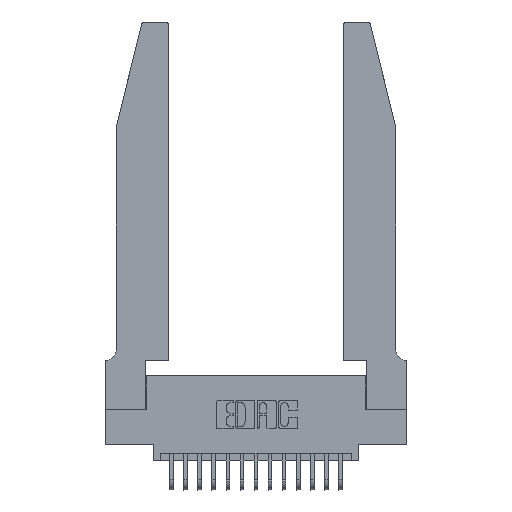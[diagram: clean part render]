
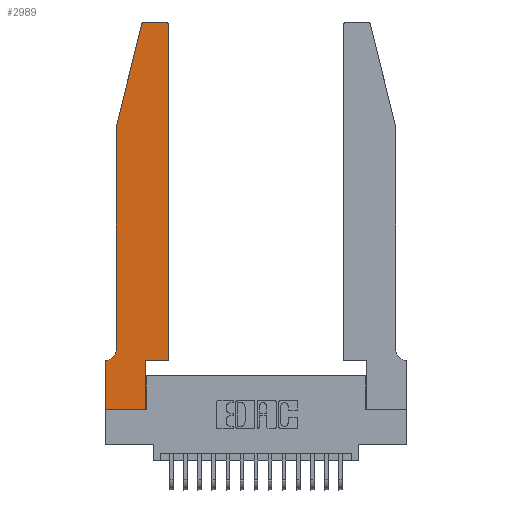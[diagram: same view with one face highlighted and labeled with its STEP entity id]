
A CAD part, top view. The second image highlights one B-rep face of the part: STEP entity #2989.
In plain terms, the highlighted planar face has unit normal (0, 0, 1).
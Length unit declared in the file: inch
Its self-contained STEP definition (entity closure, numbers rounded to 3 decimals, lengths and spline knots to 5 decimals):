
#300 = LINE ( 'NONE', #2941, #4768 ) ;
#366 = LINE ( 'NONE', #4819, #11570 ) ;
#391 = LINE ( 'NONE', #14440, #17634 ) ;
#710 = LINE ( 'NONE', #4108, #5649 ) ;
#1479 = DIRECTION ( 'NONE',  ( -1., 0., 0. ) ) ;
#1482 = LINE ( 'NONE', #8714, #19167 ) ;
#1690 = ORIENTED_EDGE ( 'NONE', *, *, #13497, .T. ) ;
#1854 = ORIENTED_EDGE ( 'NONE', *, *, #9211, .T. ) ;
#1937 = VERTEX_POINT ( 'NONE', #15944 ) ;
#2210 = CARTESIAN_POINT ( 'NONE',  ( 0.2865, 0.35, 0.37 ) ) ;
#2313 = DIRECTION ( 'NONE',  ( 0., -1., 0. ) ) ;
#2351 = VECTOR ( 'NONE', #18720, 39.37008 ) ;
#2941 = CARTESIAN_POINT ( 'NONE',  ( 0.2605, 2.75, 0.37 ) ) ;
#2953 = CARTESIAN_POINT ( 'NONE',  ( 0.4505, 0.35, 0.37 ) ) ;
#2989 = ADVANCED_FACE ( 'NONE', ( #18410 ), #14381, .T. ) ;
#3049 = LINE ( 'NONE', #14063, #9528 ) ;
#3139 = VERTEX_POINT ( 'NONE', #10591 ) ;
#3178 = VERTEX_POINT ( 'NONE', #9109 ) ;
#3418 = DIRECTION ( 'NONE',  ( 0., 1., 0. ) ) ;
#3432 = DIRECTION ( 'NONE',  ( 0., 0., 1. ) ) ;
#3788 = AXIS2_PLACEMENT_3D ( 'NONE', #11000, #11078, #1479 ) ;
#3955 = VERTEX_POINT ( 'NONE', #12955 ) ;
#4045 = VERTEX_POINT ( 'NONE', #16557 ) ;
#4108 = CARTESIAN_POINT ( 'NONE',  ( 0.0755, 2., 0.37 ) ) ;
#4110 = CARTESIAN_POINT ( 'NONE',  ( 0.2865, 0., 0.37 ) ) ;
#4365 = VERTEX_POINT ( 'NONE', #2953 ) ;
#4556 = ORIENTED_EDGE ( 'NONE', *, *, #14041, .T. ) ;
#4755 = DIRECTION ( 'NONE',  ( 1., 0., 0. ) ) ;
#4761 = EDGE_CURVE ( 'NONE', #11568, #12976, #7322, .T. ) ;
#4768 = VECTOR ( 'NONE', #17329, 39.37008 ) ;
#4790 = VERTEX_POINT ( 'NONE', #2210 ) ;
#4819 = CARTESIAN_POINT ( 'NONE',  ( 0.2865, 0.35, 0.37 ) ) ;
#5649 = VECTOR ( 'NONE', #19722, 39.37008 ) ;
#5850 = CIRCLE ( 'NONE', #19916, 0.03 ) ;
#5954 = DIRECTION ( 'NONE',  ( 0., -1., 0. ) ) ;
#5991 = ORIENTED_EDGE ( 'NONE', *, *, #4761, .T. ) ;
#6377 = EDGE_CURVE ( 'NONE', #11281, #1937, #8044, .T. ) ;
#6470 = ORIENTED_EDGE ( 'NONE', *, *, #13893, .T. ) ;
#6488 = CARTESIAN_POINT ( 'NONE',  ( 0.0755, 0.35, 0.37 ) ) ;
#6612 = EDGE_CURVE ( 'NONE', #1937, #11568, #3049, .T. ) ;
#7322 = LINE ( 'NONE', #10566, #2351 ) ;
#7611 = EDGE_LOOP ( 'NONE', ( #16982, #15287, #4556, #6470, #18482, #8667, #11855, #5991, #1854, #1690, #13580, #14146 ) ) ;
#7884 = AXIS2_PLACEMENT_3D ( 'NONE', #8598, #15134, #18227 ) ;
#8044 = LINE ( 'NONE', #6488, #11791 ) ;
#8491 = CARTESIAN_POINT ( 'NONE',  ( 0., 0., 0.37 ) ) ;
#8598 = CARTESIAN_POINT ( 'NONE',  ( 0.4205, 2.72, 0.37 ) ) ;
#8667 = ORIENTED_EDGE ( 'NONE', *, *, #6377, .T. ) ;
#8714 = CARTESIAN_POINT ( 'NONE',  ( 0.0755, 2., 0.37 ) ) ;
#9109 = CARTESIAN_POINT ( 'NONE',  ( 0.0755, 2., 0.37 ) ) ;
#9183 = VECTOR ( 'NONE', #15044, 39.37008 ) ;
#9211 = EDGE_CURVE ( 'NONE', #12976, #4790, #366, .T. ) ;
#9447 = LINE ( 'NONE', #11898, #9183 ) ;
#9528 = VECTOR ( 'NONE', #5954, 39.37008 ) ;
#10566 = CARTESIAN_POINT ( 'NONE',  ( 0., 0., 0.37 ) ) ;
#10591 = CARTESIAN_POINT ( 'NONE',  ( 0.0755, 0.42, 0.37 ) ) ;
#11000 = CARTESIAN_POINT ( 'NONE',  ( 0.0055, 0.42, 0.37 ) ) ;
#11078 = DIRECTION ( 'NONE',  ( 0., 0., -1. ) ) ;
#11281 = VERTEX_POINT ( 'NONE', #18889 ) ;
#11568 = VERTEX_POINT ( 'NONE', #8491 ) ;
#11570 = VECTOR ( 'NONE', #17330, 39.37008 ) ;
#11791 = VECTOR ( 'NONE', #16007, 39.37008 ) ;
#11855 = ORIENTED_EDGE ( 'NONE', *, *, #6612, .T. ) ;
#11898 = CARTESIAN_POINT ( 'NONE',  ( 0.4505, 0.35, 0.37 ) ) ;
#12955 = CARTESIAN_POINT ( 'NONE',  ( 0.284, 2.75, 0.37 ) ) ;
#12976 = VERTEX_POINT ( 'NONE', #4110 ) ;
#13145 = VERTEX_POINT ( 'NONE', #20499 ) ;
#13469 = CIRCLE ( 'NONE', #3788, 0.07 ) ;
#13497 = EDGE_CURVE ( 'NONE', #4790, #4365, #9447, .T. ) ;
#13580 = ORIENTED_EDGE ( 'NONE', *, *, #15528, .T. ) ;
#13792 = VERTEX_POINT ( 'NONE', #18867 ) ;
#13893 = EDGE_CURVE ( 'NONE', #3178, #3139, #1482, .T. ) ;
#14011 = EDGE_CURVE ( 'NONE', #13145, #13792, #16651, .T. ) ;
#14041 = EDGE_CURVE ( 'NONE', #4045, #3178, #710, .T. ) ;
#14063 = CARTESIAN_POINT ( 'NONE',  ( 0., 0., 0.37 ) ) ;
#14146 = ORIENTED_EDGE ( 'NONE', *, *, #14011, .T. ) ;
#14381 = PLANE ( 'NONE',  #18903 ) ;
#14440 = CARTESIAN_POINT ( 'NONE',  ( 0.4505, 0.35, 0.37 ) ) ;
#14804 = CARTESIAN_POINT ( 'NONE',  ( 0.284, 2.72, 0.37 ) ) ;
#15044 = DIRECTION ( 'NONE',  ( 1., 0., 0. ) ) ;
#15134 = DIRECTION ( 'NONE',  ( 0., 0., 1. ) ) ;
#15287 = ORIENTED_EDGE ( 'NONE', *, *, #15322, .T. ) ;
#15322 = EDGE_CURVE ( 'NONE', #3955, #4045, #5850, .T. ) ;
#15528 = EDGE_CURVE ( 'NONE', #4365, #13145, #391, .T. ) ;
#15944 = CARTESIAN_POINT ( 'NONE',  ( 0., 0.35, 0.37 ) ) ;
#16002 = CARTESIAN_POINT ( 'NONE',  ( 0., 0.35, 0.37 ) ) ;
#16007 = DIRECTION ( 'NONE',  ( -1., 0., 0. ) ) ;
#16557 = CARTESIAN_POINT ( 'NONE',  ( 0.25487, 2.72718, 0.37 ) ) ;
#16651 = CIRCLE ( 'NONE', #7884, 0.03 ) ;
#16982 = ORIENTED_EDGE ( 'NONE', *, *, #17636, .T. ) ;
#17329 = DIRECTION ( 'NONE',  ( -1., 0., 0. ) ) ;
#17330 = DIRECTION ( 'NONE',  ( 0., 1., 0. ) ) ;
#17634 = VECTOR ( 'NONE', #3418, 39.37008 ) ;
#17636 = EDGE_CURVE ( 'NONE', #13792, #3955, #300, .T. ) ;
#17891 = DIRECTION ( 'NONE',  ( 1., 0., 0. ) ) ;
#18227 = DIRECTION ( 'NONE',  ( 1., 0., 0. ) ) ;
#18291 = EDGE_CURVE ( 'NONE', #3139, #11281, #13469, .T. ) ;
#18410 = FACE_OUTER_BOUND ( 'NONE', #7611, .T. ) ;
#18482 = ORIENTED_EDGE ( 'NONE', *, *, #18291, .T. ) ;
#18720 = DIRECTION ( 'NONE',  ( 1., 0., 0. ) ) ;
#18867 = CARTESIAN_POINT ( 'NONE',  ( 0.4205, 2.75, 0.37 ) ) ;
#18889 = CARTESIAN_POINT ( 'NONE',  ( 0.0055, 0.35, 0.37 ) ) ;
#18903 = AXIS2_PLACEMENT_3D ( 'NONE', #16002, #3432, #4755 ) ;
#19167 = VECTOR ( 'NONE', #2313, 39.37008 ) ;
#19481 = DIRECTION ( 'NONE',  ( 0., 0., 1. ) ) ;
#19722 = DIRECTION ( 'NONE',  ( -0.239, -0.971, 0. ) ) ;
#19916 = AXIS2_PLACEMENT_3D ( 'NONE', #14804, #19481, #17891 ) ;
#20499 = CARTESIAN_POINT ( 'NONE',  ( 0.4505, 2.72, 0.37 ) ) ;
